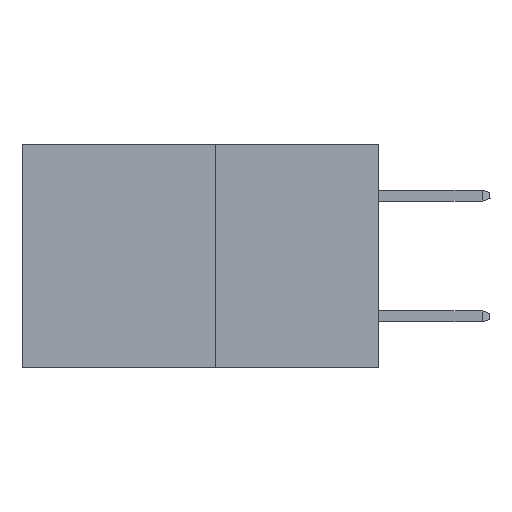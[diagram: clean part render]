
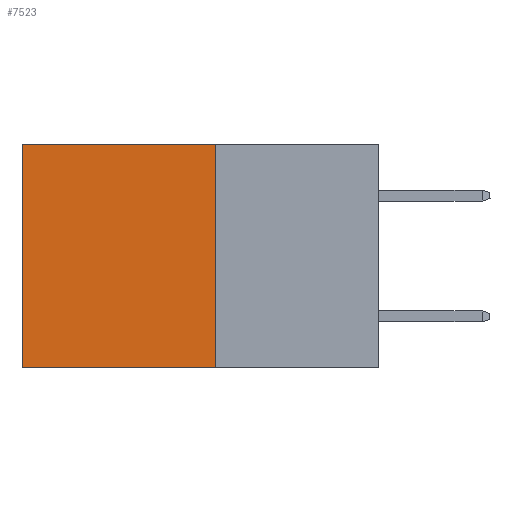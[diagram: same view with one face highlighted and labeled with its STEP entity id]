
A CAD part, left-side view. The second image highlights one B-rep face of the part: STEP entity #7523.
In plain terms, the highlighted planar face has unit normal (-1, 0, 0).
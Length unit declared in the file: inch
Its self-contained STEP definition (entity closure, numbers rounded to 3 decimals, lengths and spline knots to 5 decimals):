
#69 = ORIENTED_EDGE ( 'NONE', *, *, #2678, .F. ) ;
#212 = AXIS2_PLACEMENT_3D ( 'NONE', #18639, #17658, #17650 ) ;
#1687 = VERTEX_POINT ( 'NONE', #3198 ) ;
#2678 = EDGE_CURVE ( 'NONE', #4578, #19001, #16117, .T. ) ;
#3198 = CARTESIAN_POINT ( 'NONE',  ( 0.277, 0.59, 0. ) ) ;
#4378 = CARTESIAN_POINT ( 'NONE',  ( 0.277, 0.27, 0. ) ) ;
#4578 = VERTEX_POINT ( 'NONE', #20294 ) ;
#7523 = ADVANCED_FACE ( 'NONE', ( #30415 ), #18108, .F. ) ;
#8620 = CARTESIAN_POINT ( 'NONE',  ( 0.277, 0.27, -0.37 ) ) ;
#9919 = ORIENTED_EDGE ( 'NONE', *, *, #13934, .T. ) ;
#9998 = CARTESIAN_POINT ( 'NONE',  ( 0.277, 0.59, -0.37 ) ) ;
#11381 = EDGE_CURVE ( 'NONE', #1687, #19001, #31598, .T. ) ;
#11416 = CARTESIAN_POINT ( 'NONE',  ( 0.277, 0.27, -0.37 ) ) ;
#12466 = DIRECTION ( 'NONE',  ( 0., 0., -1. ) ) ;
#12845 = DIRECTION ( 'NONE',  ( 0., 1., 0. ) ) ;
#13201 = EDGE_LOOP ( 'NONE', ( #30962, #69, #19707, #9919 ) ) ;
#13934 = EDGE_CURVE ( 'NONE', #23638, #1687, #21352, .T. ) ;
#16117 = LINE ( 'NONE', #8620, #21840 ) ;
#17650 = DIRECTION ( 'NONE',  ( 0., 0., -1. ) ) ;
#17658 = DIRECTION ( 'NONE',  ( 1., 0., 0. ) ) ;
#18108 = PLANE ( 'NONE',  #212 ) ;
#18639 = CARTESIAN_POINT ( 'NONE',  ( 0.277, 0.27, -0.37 ) ) ;
#18815 = DIRECTION ( 'NONE',  ( 0., 0., -1. ) ) ;
#19001 = VERTEX_POINT ( 'NONE', #29006 ) ;
#19257 = LINE ( 'NONE', #11416, #25738 ) ;
#19707 = ORIENTED_EDGE ( 'NONE', *, *, #22227, .F. ) ;
#20294 = CARTESIAN_POINT ( 'NONE',  ( 0.277, 0.27, -0.37 ) ) ;
#20601 = VECTOR ( 'NONE', #28789, 39.37008 ) ;
#21229 = CARTESIAN_POINT ( 'NONE',  ( 0.277, 0.27, 0. ) ) ;
#21352 = LINE ( 'NONE', #4378, #20601 ) ;
#21840 = VECTOR ( 'NONE', #12845, 39.37008 ) ;
#22227 = EDGE_CURVE ( 'NONE', #23638, #4578, #19257, .T. ) ;
#23638 = VERTEX_POINT ( 'NONE', #21229 ) ;
#25738 = VECTOR ( 'NONE', #18815, 39.37008 ) ;
#26025 = VECTOR ( 'NONE', #12466, 39.37008 ) ;
#28789 = DIRECTION ( 'NONE',  ( 0., 1., 0. ) ) ;
#29006 = CARTESIAN_POINT ( 'NONE',  ( 0.277, 0.59, -0.37 ) ) ;
#30415 = FACE_OUTER_BOUND ( 'NONE', #13201, .T. ) ;
#30962 = ORIENTED_EDGE ( 'NONE', *, *, #11381, .T. ) ;
#31598 = LINE ( 'NONE', #9998, #26025 ) ;
